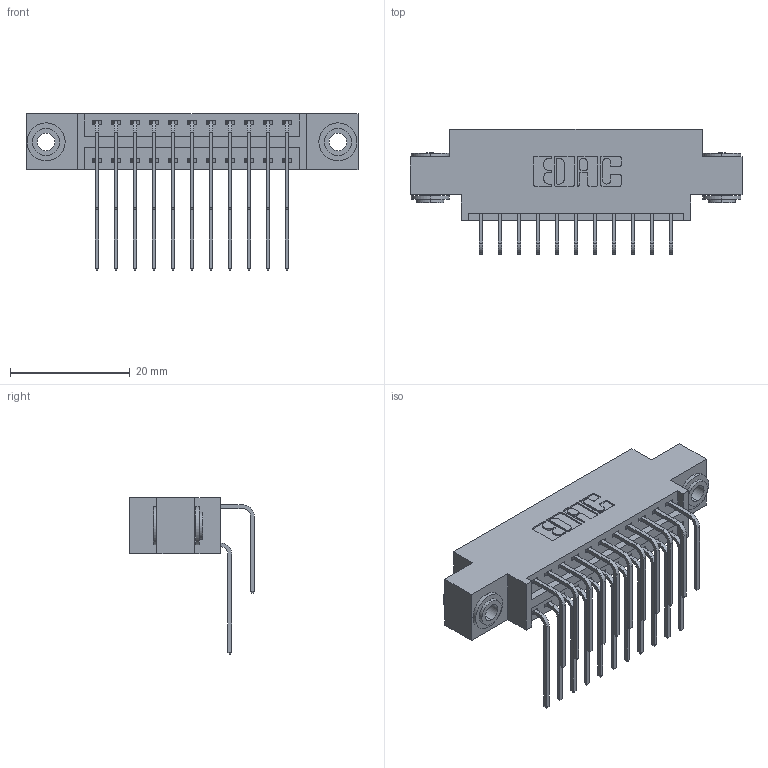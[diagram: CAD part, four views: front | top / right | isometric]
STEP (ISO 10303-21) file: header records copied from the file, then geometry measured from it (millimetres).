
FILE_DESCRIPTION (( 'STEP AP203' ), '1' );
FILE_NAME ('346-022-559-803.STEP', '2022-05-18T22:15:09', ( '' ), ( '' ), 'SwSTEP 2.0', 'SolidWorks 2020', '' );
FILE_SCHEMA (( 'CONFIG_CONTROL_DESIGN' ));
Length unit declared in the file: inch
Products named in the file (5): 346 Part_0.170 Offset - 0.156 Dia-TH; 345-292-001_558 559 Tail - 1; 346-022-559-803; 345-250-002_345-250-002-102; 345-292-001_559 Tail - 2
Assembly tree (25 placements, depth 2):
  346-022-559-803
    346 Part_0.170 Offset - 0.156 Dia-TH
    345-292-001_558 559 Tail - 1  x11
    345-292-001_559 Tail - 2  x11
    345-250-002_345-250-002-102  x2
Bounding box: 55.5 x 20.89 x 26.16 mm (x, y, z)
Volume: 5144.7 mm3; surface area: 7621.6 mm2
Topology: 25 solids, 25 shells, 1366 faces, 3995 edges, 2630 vertices
Faces by surface type: plane 918, cylinder 440, cone 8
Entity records: 14334 total; most frequent: CARTESIAN_POINT 2440, ORIENTED_EDGE 2314, DIRECTION 2203, EDGE_CURVE 1157, LINE 917, VECTOR 917, VERTEX_POINT 766, AXIS2_PLACEMENT_3D 643
